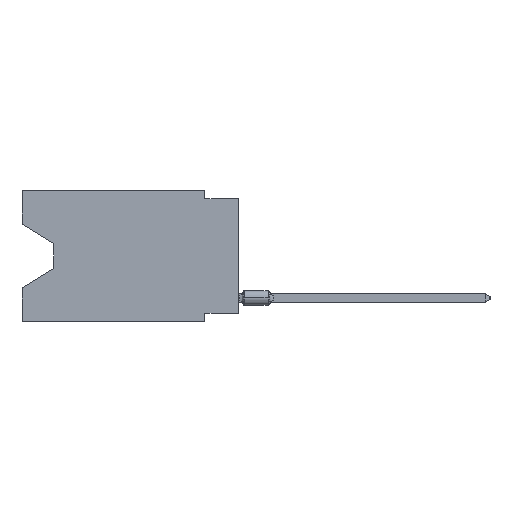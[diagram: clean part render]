
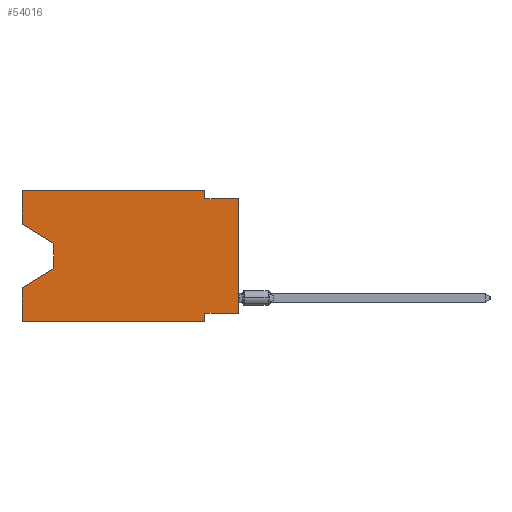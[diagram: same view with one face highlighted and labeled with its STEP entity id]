
A CAD part, left-side view. The second image highlights one B-rep face of the part: STEP entity #54016.
In plain terms, the highlighted planar face has unit normal (-1, 0, 0).
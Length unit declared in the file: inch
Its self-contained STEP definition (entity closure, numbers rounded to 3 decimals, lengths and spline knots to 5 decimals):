
#230 = VERTEX_POINT ( 'NONE', #42728 ) ;
#3050 = EDGE_CURVE ( 'NONE', #230, #65255, #77364, .T. ) ;
#4423 = EDGE_LOOP ( 'NONE', ( #81850, #40992, #76484, #19552, #7156, #23902, #17193, #38021, #79525, #23730, #23007, #45391 ) ) ;
#4768 = EDGE_CURVE ( 'NONE', #69557, #43692, #57626, .T. ) ;
#7156 = ORIENTED_EDGE ( 'NONE', *, *, #69749, .T. ) ;
#7891 = LINE ( 'NONE', #41300, #49542 ) ;
#8110 = CARTESIAN_POINT ( 'NONE',  ( 0., 0.645, -0.39 ) ) ;
#12812 = LINE ( 'NONE', #19050, #78239 ) ;
#15352 = EDGE_CURVE ( 'NONE', #52997, #78019, #28013, .T. ) ;
#16356 = CARTESIAN_POINT ( 'NONE',  ( 0., 0.55, -0.232 ) ) ;
#17193 = ORIENTED_EDGE ( 'NONE', *, *, #40157, .F. ) ;
#17270 = VECTOR ( 'NONE', #61731, 39.37008 ) ;
#17326 = FACE_OUTER_BOUND ( 'NONE', #4423, .T. ) ;
#19050 = CARTESIAN_POINT ( 'NONE',  ( 0., 0., -0.025 ) ) ;
#19496 = CARTESIAN_POINT ( 'NONE',  ( 0., 0., -0.365 ) ) ;
#19552 = ORIENTED_EDGE ( 'NONE', *, *, #20900, .F. ) ;
#20732 = VECTOR ( 'NONE', #69282, 39.37008 ) ;
#20900 = EDGE_CURVE ( 'NONE', #86018, #65255, #7891, .T. ) ;
#22958 = VECTOR ( 'NONE', #79425, 39.37008 ) ;
#23007 = ORIENTED_EDGE ( 'NONE', *, *, #85869, .F. ) ;
#23410 = CARTESIAN_POINT ( 'NONE',  ( 0., 0.1, -0.365 ) ) ;
#23478 = DIRECTION ( 'NONE',  ( 0., 0., 1. ) ) ;
#23730 = ORIENTED_EDGE ( 'NONE', *, *, #15352, .F. ) ;
#23902 = ORIENTED_EDGE ( 'NONE', *, *, #50323, .F. ) ;
#23996 = DIRECTION ( 'NONE',  ( 0., 0., -1. ) ) ;
#24075 = LINE ( 'NONE', #78423, #81595 ) ;
#24898 = DIRECTION ( 'NONE',  ( 0., 0., -1. ) ) ;
#25903 = VECTOR ( 'NONE', #87521, 39.37008 ) ;
#26395 = LINE ( 'NONE', #78973, #22958 ) ;
#28013 = LINE ( 'NONE', #55167, #38539 ) ;
#30172 = LINE ( 'NONE', #57752, #61149 ) ;
#30245 = DIRECTION ( 'NONE',  ( 1., 0., 0. ) ) ;
#31683 = VERTEX_POINT ( 'NONE', #39050 ) ;
#34588 = LINE ( 'NONE', #55492, #17270 ) ;
#35049 = DIRECTION ( 'NONE',  ( 0., 0., 1. ) ) ;
#35973 = CARTESIAN_POINT ( 'NONE',  ( 0., 0.645, 0. ) ) ;
#36777 = VECTOR ( 'NONE', #24898, 39.37008 ) ;
#38021 = ORIENTED_EDGE ( 'NONE', *, *, #4768, .T. ) ;
#38539 = VECTOR ( 'NONE', #82374, 39.37008 ) ;
#38959 = LINE ( 'NONE', #66098, #25903 ) ;
#39050 = CARTESIAN_POINT ( 'NONE',  ( 0., 0.645, -0.10025 ) ) ;
#39880 = VERTEX_POINT ( 'NONE', #75093 ) ;
#40157 = EDGE_CURVE ( 'NONE', #69557, #50466, #38959, .T. ) ;
#40992 = ORIENTED_EDGE ( 'NONE', *, *, #78419, .T. ) ;
#41300 = CARTESIAN_POINT ( 'NONE',  ( 0., 0.645, 0. ) ) ;
#42019 = EDGE_CURVE ( 'NONE', #31683, #83267, #24075, .T. ) ;
#42728 = CARTESIAN_POINT ( 'NONE',  ( 0., 0.55, -0.232 ) ) ;
#43692 = VERTEX_POINT ( 'NONE', #48019 ) ;
#45391 = ORIENTED_EDGE ( 'NONE', *, *, #82423, .F. ) ;
#45801 = CARTESIAN_POINT ( 'NONE',  ( 0., 0.1, 0. ) ) ;
#47782 = CARTESIAN_POINT ( 'NONE',  ( 0., 0.645, -0.28975 ) ) ;
#48019 = CARTESIAN_POINT ( 'NONE',  ( 0., 0., -0.025 ) ) ;
#49542 = VECTOR ( 'NONE', #35049, 39.37008 ) ;
#49745 = VECTOR ( 'NONE', #70680, 39.37008 ) ;
#50323 = EDGE_CURVE ( 'NONE', #50466, #39880, #76864, .T. ) ;
#50348 = DIRECTION ( 'NONE',  ( 0., -0.855, -0.519 ) ) ;
#50466 = VERTEX_POINT ( 'NONE', #23410 ) ;
#50699 = CARTESIAN_POINT ( 'NONE',  ( 0., 0.645, 0. ) ) ;
#51386 = DIRECTION ( 'NONE',  ( 0., 0., 1. ) ) ;
#52462 = PLANE ( 'NONE',  #88109 ) ;
#52997 = VERTEX_POINT ( 'NONE', #45801 ) ;
#54016 = ADVANCED_FACE ( 'NONE', ( #17326 ), #52462, .F. ) ;
#55167 = CARTESIAN_POINT ( 'NONE',  ( 0., 0.1, 0. ) ) ;
#55492 = CARTESIAN_POINT ( 'NONE',  ( 0., 0.645, -0.39 ) ) ;
#57626 = LINE ( 'NONE', #63871, #78745 ) ;
#57752 = CARTESIAN_POINT ( 'NONE',  ( 0., 0.645, 0. ) ) ;
#59727 = CARTESIAN_POINT ( 'NONE',  ( 0., 0.1, -0.025 ) ) ;
#61149 = VECTOR ( 'NONE', #23478, 39.37008 ) ;
#61731 = DIRECTION ( 'NONE',  ( 0., -1., 0. ) ) ;
#63871 = CARTESIAN_POINT ( 'NONE',  ( 0., 0., 0. ) ) ;
#64099 = VERTEX_POINT ( 'NONE', #35973 ) ;
#65255 = VERTEX_POINT ( 'NONE', #47782 ) ;
#66098 = CARTESIAN_POINT ( 'NONE',  ( 0., 0., -0.365 ) ) ;
#69282 = DIRECTION ( 'NONE',  ( 0., 0., -1. ) ) ;
#69514 = EDGE_CURVE ( 'NONE', #78019, #43692, #12812, .T. ) ;
#69557 = VERTEX_POINT ( 'NONE', #19496 ) ;
#69749 = EDGE_CURVE ( 'NONE', #86018, #39880, #34588, .T. ) ;
#70680 = DIRECTION ( 'NONE',  ( 0., 0.855, -0.519 ) ) ;
#74745 = CARTESIAN_POINT ( 'NONE',  ( 0., 0.55, -0.158 ) ) ;
#75093 = CARTESIAN_POINT ( 'NONE',  ( 0., 0.1, -0.39 ) ) ;
#76484 = ORIENTED_EDGE ( 'NONE', *, *, #3050, .T. ) ;
#76864 = LINE ( 'NONE', #82240, #20732 ) ;
#77364 = LINE ( 'NONE', #16356, #49745 ) ;
#78019 = VERTEX_POINT ( 'NONE', #59727 ) ;
#78239 = VECTOR ( 'NONE', #88106, 39.37008 ) ;
#78419 = EDGE_CURVE ( 'NONE', #83267, #230, #79251, .T. ) ;
#78423 = CARTESIAN_POINT ( 'NONE',  ( 0., 0.645, -0.10025 ) ) ;
#78745 = VECTOR ( 'NONE', #51386, 39.37008 ) ;
#78973 = CARTESIAN_POINT ( 'NONE',  ( 0., 0.645, 0. ) ) ;
#79251 = LINE ( 'NONE', #85059, #36777 ) ;
#79425 = DIRECTION ( 'NONE',  ( 0., -1., 0. ) ) ;
#79525 = ORIENTED_EDGE ( 'NONE', *, *, #69514, .F. ) ;
#81595 = VECTOR ( 'NONE', #50348, 39.37008 ) ;
#81850 = ORIENTED_EDGE ( 'NONE', *, *, #42019, .T. ) ;
#82240 = CARTESIAN_POINT ( 'NONE',  ( 0., 0.1, -0.39 ) ) ;
#82374 = DIRECTION ( 'NONE',  ( 0., 0., -1. ) ) ;
#82423 = EDGE_CURVE ( 'NONE', #31683, #64099, #30172, .T. ) ;
#83267 = VERTEX_POINT ( 'NONE', #74745 ) ;
#85059 = CARTESIAN_POINT ( 'NONE',  ( 0., 0.55, -0.158 ) ) ;
#85869 = EDGE_CURVE ( 'NONE', #64099, #52997, #26395, .T. ) ;
#86018 = VERTEX_POINT ( 'NONE', #8110 ) ;
#87521 = DIRECTION ( 'NONE',  ( 0., 1., 0. ) ) ;
#88106 = DIRECTION ( 'NONE',  ( 0., -1., 0. ) ) ;
#88109 = AXIS2_PLACEMENT_3D ( 'NONE', #50699, #30245, #23996 ) ;
